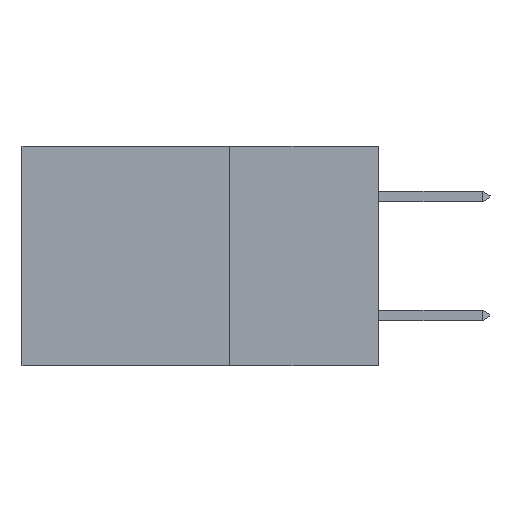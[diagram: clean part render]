
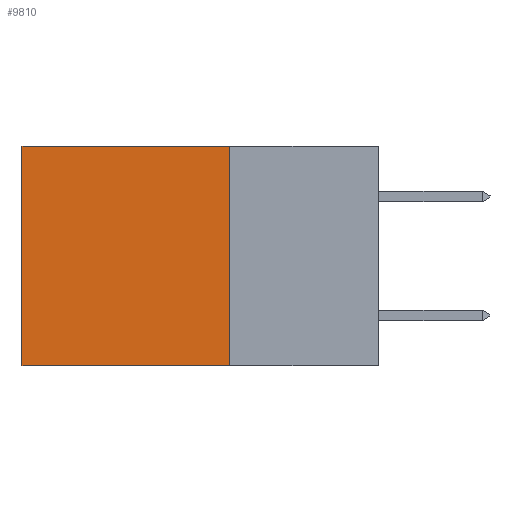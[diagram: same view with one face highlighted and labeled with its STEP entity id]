
A CAD part, left-side view. The second image highlights one B-rep face of the part: STEP entity #9810.
In plain terms, the highlighted planar face has unit normal (-1, 0, 0).
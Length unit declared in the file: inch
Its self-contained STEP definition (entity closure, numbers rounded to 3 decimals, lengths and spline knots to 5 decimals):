
#733 = VERTEX_POINT ( 'NONE', #11556 ) ;
#1123 = FACE_OUTER_BOUND ( 'NONE', #12817, .T. ) ;
#1323 = DIRECTION ( 'NONE',  ( 0., 0., -1. ) ) ;
#1868 = VERTEX_POINT ( 'NONE', #8519 ) ;
#1885 = DIRECTION ( 'NONE',  ( 0., 1., 0. ) ) ;
#1891 = EDGE_CURVE ( 'NONE', #16139, #5713, #10005, .T. ) ;
#2953 = DIRECTION ( 'NONE',  ( 0., 1., 0. ) ) ;
#3130 = CARTESIAN_POINT ( 'NONE',  ( 0.2615, 0.25, 0. ) ) ;
#3169 = ORIENTED_EDGE ( 'NONE', *, *, #11411, .T. ) ;
#4531 = EDGE_CURVE ( 'NONE', #5713, #1868, #14333, .T. ) ;
#5713 = VERTEX_POINT ( 'NONE', #13189 ) ;
#6292 = VECTOR ( 'NONE', #1885, 39.37008 ) ;
#6840 = CARTESIAN_POINT ( 'NONE',  ( 0.2615, 0.25, -0.37 ) ) ;
#7331 = LINE ( 'NONE', #12987, #6292 ) ;
#8444 = CARTESIAN_POINT ( 'NONE',  ( 0.2615, 0.6, -0.37 ) ) ;
#8519 = CARTESIAN_POINT ( 'NONE',  ( 0.2615, 0.6, -0.37 ) ) ;
#8610 = DIRECTION ( 'NONE',  ( 0., 0., -1. ) ) ;
#8665 = ORIENTED_EDGE ( 'NONE', *, *, #12278, .T. ) ;
#8850 = VECTOR ( 'NONE', #8610, 39.37008 ) ;
#9286 = ORIENTED_EDGE ( 'NONE', *, *, #1891, .F. ) ;
#9750 = LINE ( 'NONE', #8444, #16086 ) ;
#9810 = ADVANCED_FACE ( 'NONE', ( #1123 ), #18105, .F. ) ;
#10005 = LINE ( 'NONE', #15683, #8850 ) ;
#10862 = DIRECTION ( 'NONE',  ( 1., 0., 0. ) ) ;
#11411 = EDGE_CURVE ( 'NONE', #16139, #733, #7331, .T. ) ;
#11556 = CARTESIAN_POINT ( 'NONE',  ( 0.2615, 0.6, 0. ) ) ;
#12278 = EDGE_CURVE ( 'NONE', #733, #1868, #9750, .T. ) ;
#12516 = DIRECTION ( 'NONE',  ( 0., 0., -1. ) ) ;
#12817 = EDGE_LOOP ( 'NONE', ( #8665, #15692, #9286, #3169 ) ) ;
#12987 = CARTESIAN_POINT ( 'NONE',  ( 0.2615, 0.25, 0. ) ) ;
#13189 = CARTESIAN_POINT ( 'NONE',  ( 0.2615, 0.25, -0.37 ) ) ;
#13346 = VECTOR ( 'NONE', #2953, 39.37008 ) ;
#14333 = LINE ( 'NONE', #17042, #13346 ) ;
#15683 = CARTESIAN_POINT ( 'NONE',  ( 0.2615, 0.25, -0.37 ) ) ;
#15692 = ORIENTED_EDGE ( 'NONE', *, *, #4531, .F. ) ;
#16086 = VECTOR ( 'NONE', #1323, 39.37008 ) ;
#16139 = VERTEX_POINT ( 'NONE', #3130 ) ;
#17042 = CARTESIAN_POINT ( 'NONE',  ( 0.2615, 0.25, -0.37 ) ) ;
#17857 = AXIS2_PLACEMENT_3D ( 'NONE', #6840, #10862, #12516 ) ;
#18105 = PLANE ( 'NONE',  #17857 ) ;
